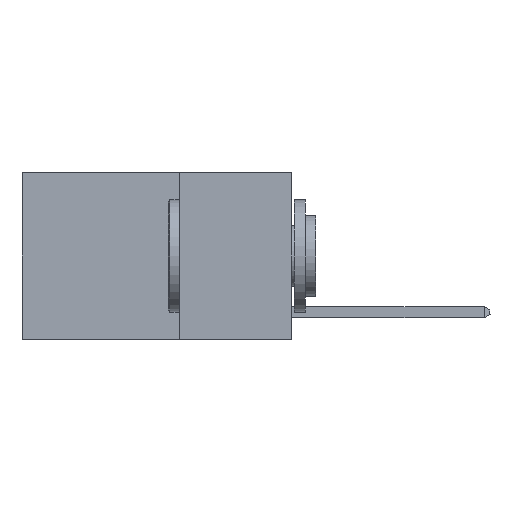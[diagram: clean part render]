
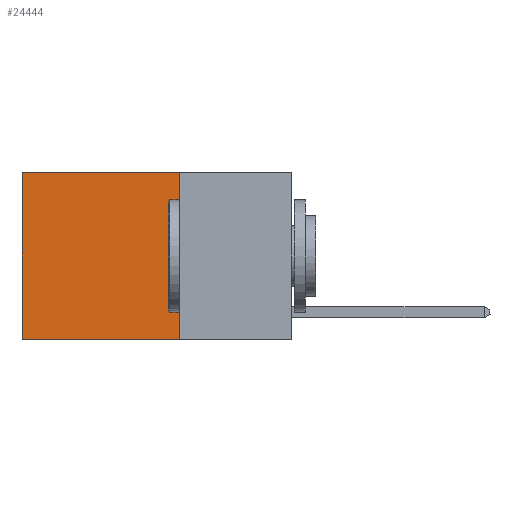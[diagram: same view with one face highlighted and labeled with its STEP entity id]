
A CAD part, left-side view. The second image highlights one B-rep face of the part: STEP entity #24444.
In plain terms, the highlighted planar face has unit normal (-1, 0, 0).
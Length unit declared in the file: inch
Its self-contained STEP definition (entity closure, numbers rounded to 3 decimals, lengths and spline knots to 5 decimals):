
#531 = LINE ( 'NONE', #25420, #24978 ) ;
#1131 = DIRECTION ( 'NONE',  ( 0., 0., -1. ) ) ;
#2770 = DIRECTION ( 'NONE',  ( 0., 1., 0. ) ) ;
#5175 = CARTESIAN_POINT ( 'NONE',  ( 0.2625, 0.25, -0.37 ) ) ;
#5878 = VERTEX_POINT ( 'NONE', #24199 ) ;
#7526 = CARTESIAN_POINT ( 'NONE',  ( 0.2625, 0.6, -0.37 ) ) ;
#8362 = EDGE_CURVE ( 'NONE', #5878, #14987, #11168, .T. ) ;
#8899 = DIRECTION ( 'NONE',  ( 0., 0., -1. ) ) ;
#9239 = CARTESIAN_POINT ( 'NONE',  ( 0.2625, 0.25, 0. ) ) ;
#9501 = VECTOR ( 'NONE', #19279, 39.37008 ) ;
#11168 = LINE ( 'NONE', #17742, #11562 ) ;
#11293 = FACE_OUTER_BOUND ( 'NONE', #15133, .T. ) ;
#11436 = PLANE ( 'NONE',  #24096 ) ;
#11562 = VECTOR ( 'NONE', #21618, 39.37008 ) ;
#12891 = VERTEX_POINT ( 'NONE', #7526 ) ;
#14987 = VERTEX_POINT ( 'NONE', #5175 ) ;
#15020 = LINE ( 'NONE', #23427, #9501 ) ;
#15133 = EDGE_LOOP ( 'NONE', ( #23566, #22986, #25754, #26785 ) ) ;
#17503 = EDGE_CURVE ( 'NONE', #5878, #18094, #21208, .T. ) ;
#17742 = CARTESIAN_POINT ( 'NONE',  ( 0.2625, 0.25, 0. ) ) ;
#17876 = DIRECTION ( 'NONE',  ( 1., 0., 0. ) ) ;
#18094 = VERTEX_POINT ( 'NONE', #20202 ) ;
#19279 = DIRECTION ( 'NONE',  ( 0., 1., 0. ) ) ;
#19814 = CARTESIAN_POINT ( 'NONE',  ( 0.2625, 0.25, 0. ) ) ;
#20202 = CARTESIAN_POINT ( 'NONE',  ( 0.2625, 0.6, 0. ) ) ;
#21208 = LINE ( 'NONE', #9239, #21461 ) ;
#21461 = VECTOR ( 'NONE', #2770, 39.37008 ) ;
#21618 = DIRECTION ( 'NONE',  ( 0., 0., -1. ) ) ;
#22271 = EDGE_CURVE ( 'NONE', #14987, #12891, #15020, .T. ) ;
#22986 = ORIENTED_EDGE ( 'NONE', *, *, #22271, .F. ) ;
#23427 = CARTESIAN_POINT ( 'NONE',  ( 0.2625, 0.25, -0.37 ) ) ;
#23566 = ORIENTED_EDGE ( 'NONE', *, *, #26406, .T. ) ;
#24096 = AXIS2_PLACEMENT_3D ( 'NONE', #19814, #17876, #1131 ) ;
#24199 = CARTESIAN_POINT ( 'NONE',  ( 0.2625, 0.25, 0. ) ) ;
#24444 = ADVANCED_FACE ( 'NONE', ( #11293 ), #11436, .F. ) ;
#24978 = VECTOR ( 'NONE', #8899, 39.37008 ) ;
#25420 = CARTESIAN_POINT ( 'NONE',  ( 0.2625, 0.6, 0. ) ) ;
#25754 = ORIENTED_EDGE ( 'NONE', *, *, #8362, .F. ) ;
#26406 = EDGE_CURVE ( 'NONE', #18094, #12891, #531, .T. ) ;
#26785 = ORIENTED_EDGE ( 'NONE', *, *, #17503, .T. ) ;
